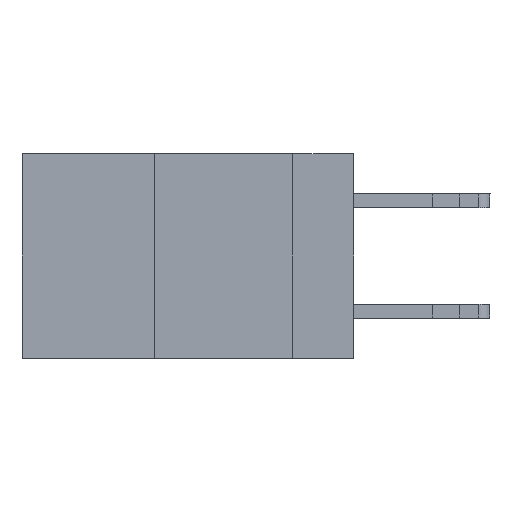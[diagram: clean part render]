
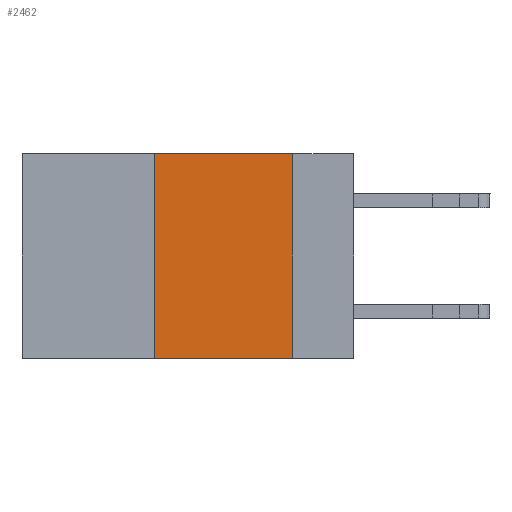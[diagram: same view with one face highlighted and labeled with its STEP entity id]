
A CAD part, left-side view. The second image highlights one B-rep face of the part: STEP entity #2462.
In plain terms, the highlighted planar face has unit normal (-1, 0, 0).
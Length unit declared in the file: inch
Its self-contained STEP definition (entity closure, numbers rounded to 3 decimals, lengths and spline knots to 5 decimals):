
#268 = EDGE_CURVE ( 'NONE', #15731, #977, #3937, .T. ) ;
#476 = CARTESIAN_POINT ( 'NONE',  ( 0., 0.11, 0. ) ) ;
#976 = ORIENTED_EDGE ( 'NONE', *, *, #14220, .F. ) ;
#977 = VERTEX_POINT ( 'NONE', #476 ) ;
#1487 = EDGE_LOOP ( 'NONE', ( #2201, #19078, #976, #4152 ) ) ;
#2201 = ORIENTED_EDGE ( 'NONE', *, *, #9717, .F. ) ;
#2462 = ADVANCED_FACE ( 'NONE', ( #5710 ), #11927, .F. ) ;
#2572 = EDGE_CURVE ( 'NONE', #12320, #14022, #4519, .T. ) ;
#2770 = CARTESIAN_POINT ( 'NONE',  ( 0., 0.36, 0. ) ) ;
#3937 = LINE ( 'NONE', #10598, #9039 ) ;
#3987 = LINE ( 'NONE', #4980, #17257 ) ;
#4152 = ORIENTED_EDGE ( 'NONE', *, *, #2572, .T. ) ;
#4519 = LINE ( 'NONE', #16083, #15901 ) ;
#4647 = AXIS2_PLACEMENT_3D ( 'NONE', #14916, #12431, #6425 ) ;
#4980 = CARTESIAN_POINT ( 'NONE',  ( 0., 0.11, 0. ) ) ;
#5710 = FACE_OUTER_BOUND ( 'NONE', #1487, .T. ) ;
#6289 = CARTESIAN_POINT ( 'NONE',  ( 0., 0.36, -0.37 ) ) ;
#6425 = DIRECTION ( 'NONE',  ( 0., 0., -1. ) ) ;
#6499 = DIRECTION ( 'NONE',  ( 0., -1., 0. ) ) ;
#7128 = CARTESIAN_POINT ( 'NONE',  ( 0., 0.36, 0. ) ) ;
#9039 = VECTOR ( 'NONE', #6499, 39.37008 ) ;
#9073 = DIRECTION ( 'NONE',  ( 0., 0., 1. ) ) ;
#9717 = EDGE_CURVE ( 'NONE', #977, #14022, #3987, .T. ) ;
#10598 = CARTESIAN_POINT ( 'NONE',  ( 0., 0.6, 0. ) ) ;
#11927 = PLANE ( 'NONE',  #4647 ) ;
#12320 = VERTEX_POINT ( 'NONE', #6289 ) ;
#12431 = DIRECTION ( 'NONE',  ( 1., 0., 0. ) ) ;
#13766 = LINE ( 'NONE', #7128, #13982 ) ;
#13982 = VECTOR ( 'NONE', #9073, 39.37008 ) ;
#14022 = VERTEX_POINT ( 'NONE', #16819 ) ;
#14220 = EDGE_CURVE ( 'NONE', #12320, #15731, #13766, .T. ) ;
#14916 = CARTESIAN_POINT ( 'NONE',  ( 0., 0.6, 0. ) ) ;
#15731 = VERTEX_POINT ( 'NONE', #2770 ) ;
#15901 = VECTOR ( 'NONE', #17420, 39.37008 ) ;
#16083 = CARTESIAN_POINT ( 'NONE',  ( 0., 0.6, -0.37 ) ) ;
#16711 = DIRECTION ( 'NONE',  ( 0., 0., -1. ) ) ;
#16819 = CARTESIAN_POINT ( 'NONE',  ( 0., 0.11, -0.37 ) ) ;
#17257 = VECTOR ( 'NONE', #16711, 39.37008 ) ;
#17420 = DIRECTION ( 'NONE',  ( 0., -1., 0. ) ) ;
#19078 = ORIENTED_EDGE ( 'NONE', *, *, #268, .F. ) ;
